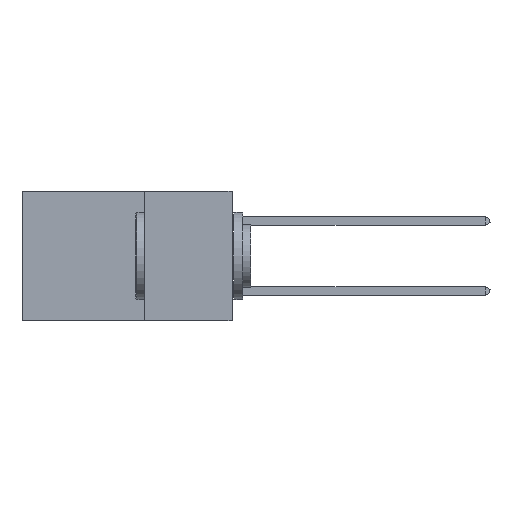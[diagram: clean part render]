
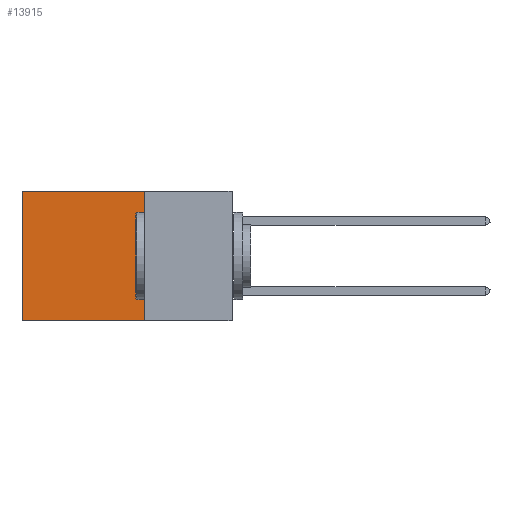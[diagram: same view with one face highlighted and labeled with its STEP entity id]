
A CAD part, left-side view. The second image highlights one B-rep face of the part: STEP entity #13915.
In plain terms, the highlighted planar face has unit normal (-1, 0, 0).
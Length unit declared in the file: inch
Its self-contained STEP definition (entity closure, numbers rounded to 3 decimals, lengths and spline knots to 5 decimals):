
#688 = CARTESIAN_POINT ( 'NONE',  ( 0.2875, 0.25, 0. ) ) ;
#2415 = DIRECTION ( 'NONE',  ( 0., 1., 0. ) ) ;
#2795 = ORIENTED_EDGE ( 'NONE', *, *, #2854, .T. ) ;
#2854 = EDGE_CURVE ( 'NONE', #31057, #22193, #25332, .T. ) ;
#5550 = CARTESIAN_POINT ( 'NONE',  ( 0.2875, 0.25, 0. ) ) ;
#6683 = DIRECTION ( 'NONE',  ( 0., 0., -1. ) ) ;
#7417 = CARTESIAN_POINT ( 'NONE',  ( 0.2875, 0.6, -0.37 ) ) ;
#10377 = VECTOR ( 'NONE', #15095, 39.37008 ) ;
#13915 = ADVANCED_FACE ( 'NONE', ( #19635 ), #21170, .F. ) ;
#14043 = EDGE_CURVE ( 'NONE', #20115, #22193, #21828, .T. ) ;
#14175 = VECTOR ( 'NONE', #2415, 39.37008 ) ;
#15095 = DIRECTION ( 'NONE',  ( 0., 0., -1. ) ) ;
#16893 = ORIENTED_EDGE ( 'NONE', *, *, #29857, .T. ) ;
#17786 = VECTOR ( 'NONE', #25437, 39.37008 ) ;
#17999 = AXIS2_PLACEMENT_3D ( 'NONE', #688, #23985, #6683 ) ;
#18368 = EDGE_CURVE ( 'NONE', #24439, #20115, #33152, .T. ) ;
#19292 = EDGE_LOOP ( 'NONE', ( #2795, #25293, #30504, #16893 ) ) ;
#19635 = FACE_OUTER_BOUND ( 'NONE', #19292, .T. ) ;
#20115 = VERTEX_POINT ( 'NONE', #33636 ) ;
#21170 = PLANE ( 'NONE',  #17999 ) ;
#21828 = LINE ( 'NONE', #25642, #14175 ) ;
#22193 = VERTEX_POINT ( 'NONE', #7417 ) ;
#23985 = DIRECTION ( 'NONE',  ( 1., 0., 0. ) ) ;
#24439 = VERTEX_POINT ( 'NONE', #35883 ) ;
#25293 = ORIENTED_EDGE ( 'NONE', *, *, #14043, .F. ) ;
#25332 = LINE ( 'NONE', #33863, #17786 ) ;
#25437 = DIRECTION ( 'NONE',  ( 0., 0., -1. ) ) ;
#25642 = CARTESIAN_POINT ( 'NONE',  ( 0.2875, 0.25, -0.37 ) ) ;
#27568 = VECTOR ( 'NONE', #31460, 39.37008 ) ;
#29857 = EDGE_CURVE ( 'NONE', #24439, #31057, #36009, .T. ) ;
#30504 = ORIENTED_EDGE ( 'NONE', *, *, #18368, .F. ) ;
#31057 = VERTEX_POINT ( 'NONE', #36472 ) ;
#31460 = DIRECTION ( 'NONE',  ( 0., 1., 0. ) ) ;
#33152 = LINE ( 'NONE', #34994, #10377 ) ;
#33636 = CARTESIAN_POINT ( 'NONE',  ( 0.2875, 0.25, -0.37 ) ) ;
#33863 = CARTESIAN_POINT ( 'NONE',  ( 0.2875, 0.6, 0. ) ) ;
#34994 = CARTESIAN_POINT ( 'NONE',  ( 0.2875, 0.25, 0. ) ) ;
#35883 = CARTESIAN_POINT ( 'NONE',  ( 0.2875, 0.25, 0. ) ) ;
#36009 = LINE ( 'NONE', #5550, #27568 ) ;
#36472 = CARTESIAN_POINT ( 'NONE',  ( 0.2875, 0.6, 0. ) ) ;
